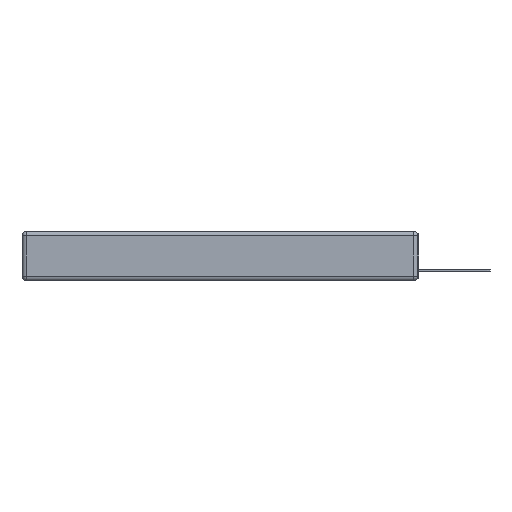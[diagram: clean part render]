
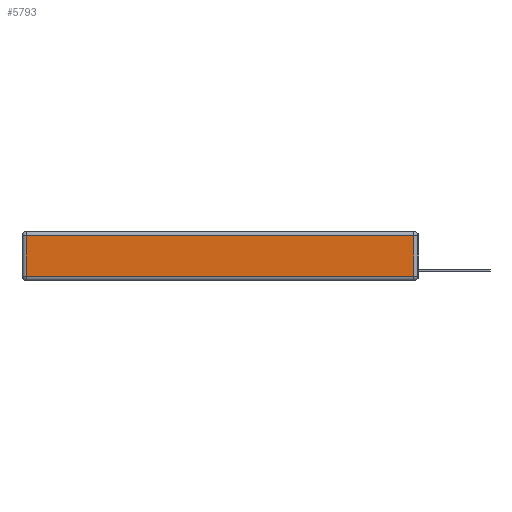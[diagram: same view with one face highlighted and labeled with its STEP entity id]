
A CAD part, left-side view. The second image highlights one B-rep face of the part: STEP entity #5793.
In plain terms, the highlighted planar face has unit normal (-1, 0, 0).
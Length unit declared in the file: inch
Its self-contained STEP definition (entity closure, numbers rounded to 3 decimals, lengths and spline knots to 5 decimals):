
#444 = EDGE_LOOP ( 'NONE', ( #6596, #24794, #21435, #2744 ) ) ;
#2744 = ORIENTED_EDGE ( 'NONE', *, *, #18902, .T. ) ;
#3667 = CARTESIAN_POINT ( 'NONE',  ( 0., 2.72, -0.343 ) ) ;
#3891 = EDGE_CURVE ( 'NONE', #8584, #15582, #16358, .T. ) ;
#3995 = VECTOR ( 'NONE', #21001, 39.37008 ) ;
#5793 = ADVANCED_FACE ( 'NONE', ( #20283 ), #9450, .T. ) ;
#6596 = ORIENTED_EDGE ( 'NONE', *, *, #3891, .T. ) ;
#6966 = VECTOR ( 'NONE', #15606, 39.37008 ) ;
#7320 = VECTOR ( 'NONE', #12921, 39.37008 ) ;
#8584 = VERTEX_POINT ( 'NONE', #17050 ) ;
#8773 = VECTOR ( 'NONE', #19191, 39.37008 ) ;
#9450 = PLANE ( 'NONE',  #13383 ) ;
#9920 = VERTEX_POINT ( 'NONE', #15084 ) ;
#10467 = CARTESIAN_POINT ( 'NONE',  ( 0., 2.72, -0.03 ) ) ;
#12921 = DIRECTION ( 'NONE',  ( 0., 1., 0. ) ) ;
#13383 = AXIS2_PLACEMENT_3D ( 'NONE', #25200, #15514, #23490 ) ;
#13857 = CARTESIAN_POINT ( 'NONE',  ( 0., 0.03, -0.343 ) ) ;
#15084 = CARTESIAN_POINT ( 'NONE',  ( 0., 0.03, -0.03 ) ) ;
#15514 = DIRECTION ( 'NONE',  ( -1., 0., 0. ) ) ;
#15582 = VERTEX_POINT ( 'NONE', #21604 ) ;
#15606 = DIRECTION ( 'NONE',  ( 0., 0., 1. ) ) ;
#15611 = EDGE_CURVE ( 'NONE', #15582, #9920, #20881, .T. ) ;
#16358 = LINE ( 'NONE', #21339, #3995 ) ;
#16899 = EDGE_CURVE ( 'NONE', #9920, #19040, #17866, .T. ) ;
#17050 = CARTESIAN_POINT ( 'NONE',  ( 0., 2.72, -0.313 ) ) ;
#17448 = CARTESIAN_POINT ( 'NONE',  ( 0., 2.75, -0.03 ) ) ;
#17778 = LINE ( 'NONE', #3667, #8773 ) ;
#17866 = LINE ( 'NONE', #17448, #7320 ) ;
#18902 = EDGE_CURVE ( 'NONE', #19040, #8584, #17778, .T. ) ;
#19040 = VERTEX_POINT ( 'NONE', #10467 ) ;
#19191 = DIRECTION ( 'NONE',  ( 0., 0., -1. ) ) ;
#20283 = FACE_OUTER_BOUND ( 'NONE', #444, .T. ) ;
#20881 = LINE ( 'NONE', #13857, #6966 ) ;
#21001 = DIRECTION ( 'NONE',  ( 0., -1., 0. ) ) ;
#21339 = CARTESIAN_POINT ( 'NONE',  ( 0., 0., -0.313 ) ) ;
#21435 = ORIENTED_EDGE ( 'NONE', *, *, #16899, .T. ) ;
#21604 = CARTESIAN_POINT ( 'NONE',  ( 0., 0.03, -0.313 ) ) ;
#23490 = DIRECTION ( 'NONE',  ( 0., 0., 1. ) ) ;
#24794 = ORIENTED_EDGE ( 'NONE', *, *, #15611, .T. ) ;
#25200 = CARTESIAN_POINT ( 'NONE',  ( 0., 0., -0.343 ) ) ;
